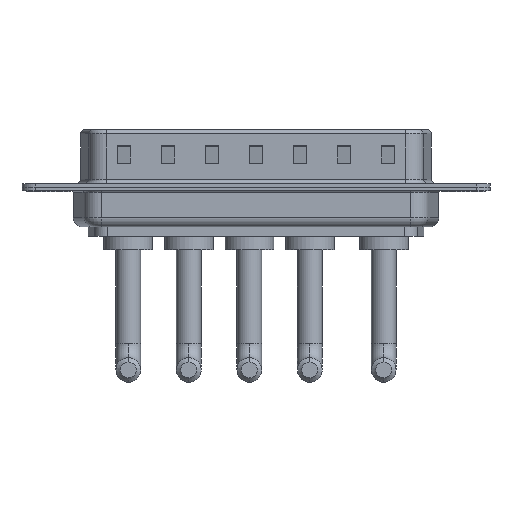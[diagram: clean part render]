
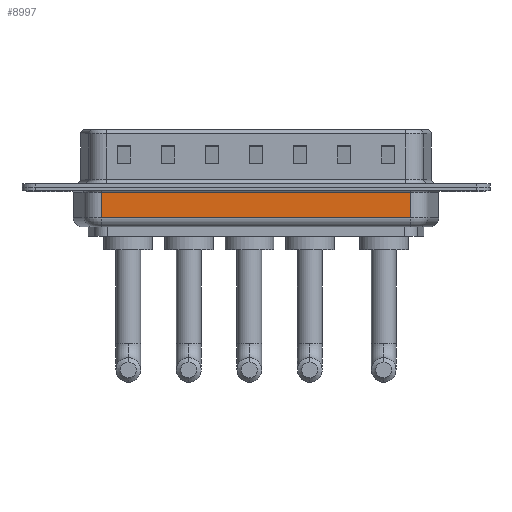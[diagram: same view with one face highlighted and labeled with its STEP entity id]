
A CAD part, front view. The second image highlights one B-rep face of the part: STEP entity #8997.
In plain terms, the highlighted planar face has unit normal (0, -1, 0).
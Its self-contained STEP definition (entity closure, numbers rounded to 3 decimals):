
#24 = CARTESIAN_POINT ( 'NONE',  ( 6.006, -5.35, -4.5 ) ) ;
#580 = DIRECTION ( 'NONE',  ( 1., 0., 0. ) ) ;
#617 = CARTESIAN_POINT ( 'NONE',  ( 41.044, -5.35, -3.5 ) ) ;
#656 = EDGE_CURVE ( 'NONE', #12021, #3332, #11602, .T. ) ;
#1730 = EDGE_LOOP ( 'NONE', ( #7920, #10285, #11159, #7168 ) ) ;
#1781 = CARTESIAN_POINT ( 'NONE',  ( 41.044, -5.35, -0.65 ) ) ;
#1850 = DIRECTION ( 'NONE',  ( -1., 0., 0. ) ) ;
#2436 = CARTESIAN_POINT ( 'NONE',  ( 6.006, -5.35, -3.5 ) ) ;
#3332 = VERTEX_POINT ( 'NONE', #11337 ) ;
#3412 = DIRECTION ( 'NONE',  ( 0., 0., 1. ) ) ;
#3855 = VECTOR ( 'NONE', #1850, 1000. ) ;
#4956 = EDGE_CURVE ( 'NONE', #12442, #12021, #12148, .T. ) ;
#5133 = VECTOR ( 'NONE', #580, 1000. ) ;
#5386 = VECTOR ( 'NONE', #12369, 1000. ) ;
#5778 = CARTESIAN_POINT ( 'NONE',  ( 6.006, -5.35, -0.65 ) ) ;
#5804 = FACE_OUTER_BOUND ( 'NONE', #1730, .T. ) ;
#5894 = VERTEX_POINT ( 'NONE', #9965 ) ;
#7168 = ORIENTED_EDGE ( 'NONE', *, *, #656, .T. ) ;
#7249 = LINE ( 'NONE', #2436, #5133 ) ;
#7426 = EDGE_CURVE ( 'NONE', #5894, #3332, #10338, .T. ) ;
#7920 = ORIENTED_EDGE ( 'NONE', *, *, #7426, .F. ) ;
#8476 = CARTESIAN_POINT ( 'NONE',  ( 6.006, -5.35, -4.5 ) ) ;
#8743 = PLANE ( 'NONE',  #12383 ) ;
#8997 = ADVANCED_FACE ( 'NONE', ( #5804 ), #8743, .F. ) ;
#9043 = DIRECTION ( 'NONE',  ( 0., 0., 1. ) ) ;
#9965 = CARTESIAN_POINT ( 'NONE',  ( 6.006, -5.35, -3.5 ) ) ;
#10236 = CARTESIAN_POINT ( 'NONE',  ( 41.044, -5.35, -4.5 ) ) ;
#10285 = ORIENTED_EDGE ( 'NONE', *, *, #10409, .T. ) ;
#10338 = LINE ( 'NONE', #8476, #5386 ) ;
#10409 = EDGE_CURVE ( 'NONE', #5894, #12442, #7249, .T. ) ;
#11159 = ORIENTED_EDGE ( 'NONE', *, *, #4956, .T. ) ;
#11337 = CARTESIAN_POINT ( 'NONE',  ( 6.006, -5.35, -0.65 ) ) ;
#11602 = LINE ( 'NONE', #5778, #3855 ) ;
#12021 = VERTEX_POINT ( 'NONE', #1781 ) ;
#12095 = VECTOR ( 'NONE', #3412, 1000. ) ;
#12115 = DIRECTION ( 'NONE',  ( 0., 1., 0. ) ) ;
#12148 = LINE ( 'NONE', #10236, #12095 ) ;
#12369 = DIRECTION ( 'NONE',  ( 0., 0., 1. ) ) ;
#12383 = AXIS2_PLACEMENT_3D ( 'NONE', #24, #12115, #9043 ) ;
#12442 = VERTEX_POINT ( 'NONE', #617 ) ;
